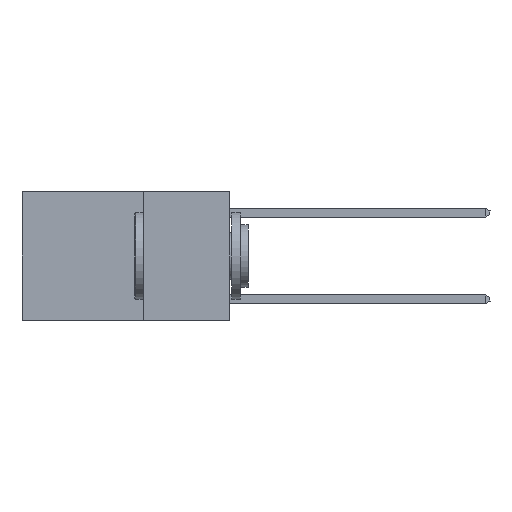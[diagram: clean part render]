
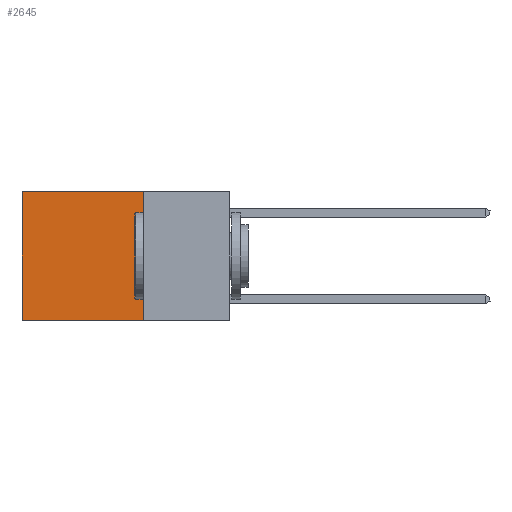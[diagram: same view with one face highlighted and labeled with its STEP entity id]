
A CAD part, left-side view. The second image highlights one B-rep face of the part: STEP entity #2645.
In plain terms, the highlighted planar face has unit normal (-1, 0, 0).
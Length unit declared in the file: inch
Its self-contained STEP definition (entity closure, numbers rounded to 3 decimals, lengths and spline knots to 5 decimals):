
#110 = LINE ( 'NONE', #9767, #5755 ) ;
#823 = VERTEX_POINT ( 'NONE', #13230 ) ;
#959 = VECTOR ( 'NONE', #2207, 39.37008 ) ;
#1000 = VERTEX_POINT ( 'NONE', #11080 ) ;
#1030 = DIRECTION ( 'NONE',  ( 0., 0., -1. ) ) ;
#1227 = EDGE_CURVE ( 'NONE', #5256, #1000, #110, .T. ) ;
#1234 = ORIENTED_EDGE ( 'NONE', *, *, #1227, .T. ) ;
#2207 = DIRECTION ( 'NONE',  ( 0., 0., -1. ) ) ;
#2220 = DIRECTION ( 'NONE',  ( 1., 0., 0. ) ) ;
#2645 = ADVANCED_FACE ( 'NONE', ( #8277 ), #13052, .F. ) ;
#2736 = VERTEX_POINT ( 'NONE', #13444 ) ;
#4209 = EDGE_CURVE ( 'NONE', #5256, #2736, #14225, .T. ) ;
#5256 = VERTEX_POINT ( 'NONE', #9522 ) ;
#5755 = VECTOR ( 'NONE', #14539, 39.37008 ) ;
#5876 = CARTESIAN_POINT ( 'NONE',  ( 0.2625, 0.25, 0. ) ) ;
#7004 = EDGE_LOOP ( 'NONE', ( #12308, #12106, #7816, #1234 ) ) ;
#7816 = ORIENTED_EDGE ( 'NONE', *, *, #4209, .F. ) ;
#8277 = FACE_OUTER_BOUND ( 'NONE', #7004, .T. ) ;
#8691 = LINE ( 'NONE', #13249, #12638 ) ;
#8901 = VECTOR ( 'NONE', #13983, 39.37008 ) ;
#9522 = CARTESIAN_POINT ( 'NONE',  ( 0.2625, 0.25, 0. ) ) ;
#9767 = CARTESIAN_POINT ( 'NONE',  ( 0.2625, 0.25, 0. ) ) ;
#10068 = CARTESIAN_POINT ( 'NONE',  ( 0.2625, 0.25, -0.37 ) ) ;
#10704 = AXIS2_PLACEMENT_3D ( 'NONE', #5876, #2220, #1030 ) ;
#10817 = DIRECTION ( 'NONE',  ( 0., 0., -1. ) ) ;
#11080 = CARTESIAN_POINT ( 'NONE',  ( 0.2625, 0.6, 0. ) ) ;
#12106 = ORIENTED_EDGE ( 'NONE', *, *, #12348, .F. ) ;
#12308 = ORIENTED_EDGE ( 'NONE', *, *, #15237, .T. ) ;
#12348 = EDGE_CURVE ( 'NONE', #2736, #823, #14927, .T. ) ;
#12638 = VECTOR ( 'NONE', #10817, 39.37008 ) ;
#13042 = CARTESIAN_POINT ( 'NONE',  ( 0.2625, 0.25, 0. ) ) ;
#13052 = PLANE ( 'NONE',  #10704 ) ;
#13230 = CARTESIAN_POINT ( 'NONE',  ( 0.2625, 0.6, -0.37 ) ) ;
#13249 = CARTESIAN_POINT ( 'NONE',  ( 0.2625, 0.6, 0. ) ) ;
#13444 = CARTESIAN_POINT ( 'NONE',  ( 0.2625, 0.25, -0.37 ) ) ;
#13983 = DIRECTION ( 'NONE',  ( 0., 1., 0. ) ) ;
#14225 = LINE ( 'NONE', #13042, #959 ) ;
#14539 = DIRECTION ( 'NONE',  ( 0., 1., 0. ) ) ;
#14927 = LINE ( 'NONE', #10068, #8901 ) ;
#15237 = EDGE_CURVE ( 'NONE', #1000, #823, #8691, .T. ) ;
